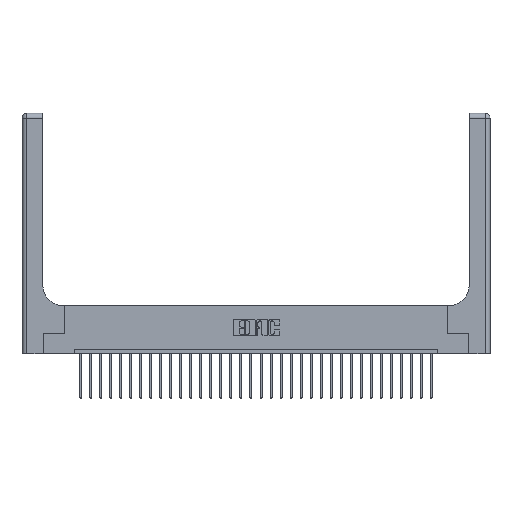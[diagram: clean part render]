
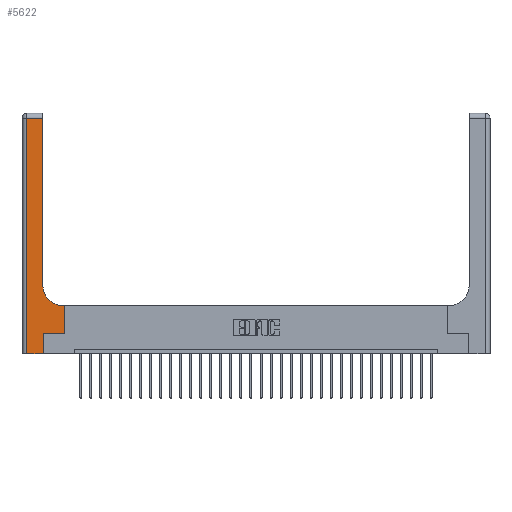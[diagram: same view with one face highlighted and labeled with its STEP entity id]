
A CAD part, top view. The second image highlights one B-rep face of the part: STEP entity #5622.
In plain terms, the highlighted planar face has unit normal (0, 0, 1).
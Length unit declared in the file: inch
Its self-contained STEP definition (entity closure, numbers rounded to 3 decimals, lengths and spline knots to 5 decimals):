
#193 = DIRECTION ( 'NONE',  ( -1., 0., 0. ) ) ;
#612 = CIRCLE ( 'NONE', #4324, 0.25 ) ;
#660 = DIRECTION ( 'NONE',  ( 0., 0., -1. ) ) ;
#753 = VERTEX_POINT ( 'NONE', #11760 ) ;
#761 = CARTESIAN_POINT ( 'NONE',  ( 0., 2.94, 0.37 ) ) ;
#952 = CARTESIAN_POINT ( 'NONE',  ( 0., 0., 0.37 ) ) ;
#1270 = LINE ( 'NONE', #23162, #21547 ) ;
#2211 = ORIENTED_EDGE ( 'NONE', *, *, #17193, .T. ) ;
#2623 = CARTESIAN_POINT ( 'NONE',  ( 0., 3., 0.37 ) ) ;
#2683 = DIRECTION ( 'NONE',  ( 0., 1., 0. ) ) ;
#2892 = DIRECTION ( 'NONE',  ( 1., 0., 0. ) ) ;
#3327 = VERTEX_POINT ( 'NONE', #23763 ) ;
#3413 = DIRECTION ( 'NONE',  ( 0., 1., 0. ) ) ;
#3843 = VECTOR ( 'NONE', #193, 39.37008 ) ;
#3976 = VECTOR ( 'NONE', #2683, 39.37008 ) ;
#4324 = AXIS2_PLACEMENT_3D ( 'NONE', #20237, #660, #16130 ) ;
#5622 = ADVANCED_FACE ( 'NONE', ( #20623 ), #24563, .F. ) ;
#5629 = ORIENTED_EDGE ( 'NONE', *, *, #14368, .T. ) ;
#5794 = ORIENTED_EDGE ( 'NONE', *, *, #9865, .T. ) ;
#6009 = VERTEX_POINT ( 'NONE', #21429 ) ;
#6920 = LINE ( 'NONE', #12260, #16927 ) ;
#7547 = DIRECTION ( 'NONE',  ( 1., 0., 0. ) ) ;
#7706 = LINE ( 'NONE', #952, #27556 ) ;
#9034 = DIRECTION ( 'NONE',  ( -1., 0., 0. ) ) ;
#9206 = LINE ( 'NONE', #14066, #27697 ) ;
#9865 = EDGE_CURVE ( 'NONE', #14201, #24352, #18483, .T. ) ;
#9916 = EDGE_CURVE ( 'NONE', #16977, #3327, #1270, .T. ) ;
#10024 = EDGE_LOOP ( 'NONE', ( #25909, #5794, #13288, #26347, #14999, #21640, #27936, #2211, #5629 ) ) ;
#10680 = CARTESIAN_POINT ( 'NONE',  ( 0.51, 0.6, 0.37 ) ) ;
#10780 = CARTESIAN_POINT ( 'NONE',  ( 0.528, 0.25, 0.37 ) ) ;
#11168 = LINE ( 'NONE', #18183, #3976 ) ;
#11760 = CARTESIAN_POINT ( 'NONE',  ( 0.528, 0.25, 0.37 ) ) ;
#12260 = CARTESIAN_POINT ( 'NONE',  ( 0.06, 3., 0.37 ) ) ;
#12683 = EDGE_CURVE ( 'NONE', #3327, #753, #9206, .T. ) ;
#12875 = LINE ( 'NONE', #10780, #20792 ) ;
#13140 = CARTESIAN_POINT ( 'NONE',  ( 0.26, 0.6, 0.37 ) ) ;
#13288 = ORIENTED_EDGE ( 'NONE', *, *, #27854, .T. ) ;
#14066 = CARTESIAN_POINT ( 'NONE',  ( 0.265, 0.25, 0.37 ) ) ;
#14201 = VERTEX_POINT ( 'NONE', #22056 ) ;
#14368 = EDGE_CURVE ( 'NONE', #15730, #19844, #612, .T. ) ;
#14999 = ORIENTED_EDGE ( 'NONE', *, *, #9916, .T. ) ;
#15403 = CARTESIAN_POINT ( 'NONE',  ( 0.06, 2.94, 0.37 ) ) ;
#15730 = VERTEX_POINT ( 'NONE', #10680 ) ;
#15812 = CARTESIAN_POINT ( 'NONE',  ( 0.265, 0., 0.37 ) ) ;
#16130 = DIRECTION ( 'NONE',  ( 1., 0., 0. ) ) ;
#16927 = VECTOR ( 'NONE', #19572, 39.37008 ) ;
#16977 = VERTEX_POINT ( 'NONE', #15812 ) ;
#17193 = EDGE_CURVE ( 'NONE', #6009, #15730, #19320, .T. ) ;
#18183 = CARTESIAN_POINT ( 'NONE',  ( 0.26, 3., 0.37 ) ) ;
#18483 = LINE ( 'NONE', #761, #22220 ) ;
#18535 = DIRECTION ( 'NONE',  ( -1., 0., 0. ) ) ;
#19320 = LINE ( 'NONE', #13140, #3843 ) ;
#19572 = DIRECTION ( 'NONE',  ( 0., -1., 0. ) ) ;
#19844 = VERTEX_POINT ( 'NONE', #23425 ) ;
#20237 = CARTESIAN_POINT ( 'NONE',  ( 0.51, 0.85, 0.37 ) ) ;
#20552 = EDGE_CURVE ( 'NONE', #19844, #14201, #11168, .T. ) ;
#20623 = FACE_OUTER_BOUND ( 'NONE', #10024, .T. ) ;
#20792 = VECTOR ( 'NONE', #28299, 39.37008 ) ;
#21429 = CARTESIAN_POINT ( 'NONE',  ( 0.528, 0.6, 0.37 ) ) ;
#21547 = VECTOR ( 'NONE', #3413, 39.37008 ) ;
#21640 = ORIENTED_EDGE ( 'NONE', *, *, #12683, .T. ) ;
#22056 = CARTESIAN_POINT ( 'NONE',  ( 0.26, 2.94, 0.37 ) ) ;
#22208 = DIRECTION ( 'NONE',  ( 0., 0., -1. ) ) ;
#22220 = VECTOR ( 'NONE', #18535, 39.37008 ) ;
#23162 = CARTESIAN_POINT ( 'NONE',  ( 0.265, 0., 0.37 ) ) ;
#23425 = CARTESIAN_POINT ( 'NONE',  ( 0.26, 0.85, 0.37 ) ) ;
#23763 = CARTESIAN_POINT ( 'NONE',  ( 0.265, 0.25, 0.37 ) ) ;
#24352 = VERTEX_POINT ( 'NONE', #15403 ) ;
#24563 = PLANE ( 'NONE',  #24925 ) ;
#24925 = AXIS2_PLACEMENT_3D ( 'NONE', #2623, #22208, #9034 ) ;
#25549 = EDGE_CURVE ( 'NONE', #27939, #16977, #7706, .T. ) ;
#25909 = ORIENTED_EDGE ( 'NONE', *, *, #20552, .T. ) ;
#26256 = EDGE_CURVE ( 'NONE', #753, #6009, #12875, .T. ) ;
#26274 = CARTESIAN_POINT ( 'NONE',  ( 0.06, 0., 0.37 ) ) ;
#26347 = ORIENTED_EDGE ( 'NONE', *, *, #25549, .T. ) ;
#27556 = VECTOR ( 'NONE', #7547, 39.37008 ) ;
#27697 = VECTOR ( 'NONE', #2892, 39.37008 ) ;
#27854 = EDGE_CURVE ( 'NONE', #24352, #27939, #6920, .T. ) ;
#27936 = ORIENTED_EDGE ( 'NONE', *, *, #26256, .T. ) ;
#27939 = VERTEX_POINT ( 'NONE', #26274 ) ;
#28299 = DIRECTION ( 'NONE',  ( 0., 1., 0. ) ) ;
